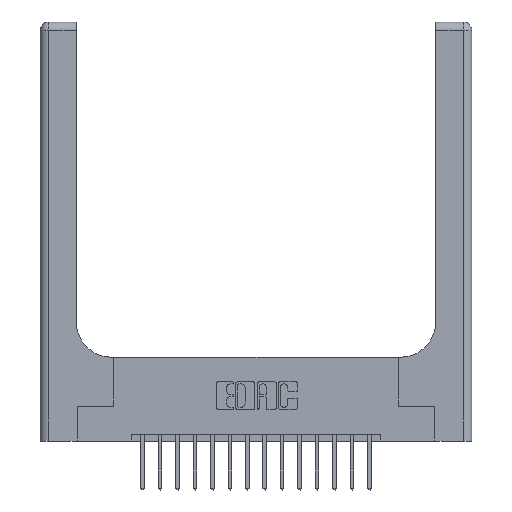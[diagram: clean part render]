
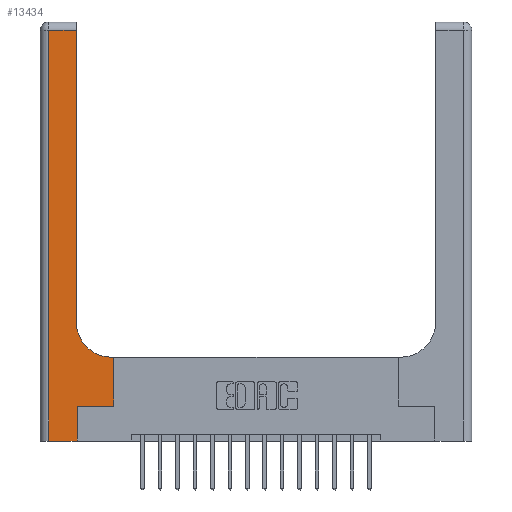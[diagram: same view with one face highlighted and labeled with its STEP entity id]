
A CAD part, top view. The second image highlights one B-rep face of the part: STEP entity #13434.
In plain terms, the highlighted planar face has unit normal (0, 0, 1).
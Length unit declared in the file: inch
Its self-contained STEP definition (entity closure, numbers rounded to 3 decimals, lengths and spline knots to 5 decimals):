
#68 = EDGE_CURVE ( 'NONE', #2373, #2701, #5165, .T. ) ;
#101 = ORIENTED_EDGE ( 'NONE', *, *, #17606, .T. ) ;
#243 = VECTOR ( 'NONE', #9647, 39.37008 ) ;
#904 = ORIENTED_EDGE ( 'NONE', *, *, #14326, .T. ) ;
#1054 = VECTOR ( 'NONE', #3244, 39.37008 ) ;
#1208 = CARTESIAN_POINT ( 'NONE',  ( 0.265, 0.25, 0.37 ) ) ;
#1668 = AXIS2_PLACEMENT_3D ( 'NONE', #18173, #14062, #3634 ) ;
#1882 = DIRECTION ( 'NONE',  ( 0., -1., 0. ) ) ;
#1957 = VERTEX_POINT ( 'NONE', #5199 ) ;
#2124 = DIRECTION ( 'NONE',  ( -1., 0., 0. ) ) ;
#2324 = CARTESIAN_POINT ( 'NONE',  ( 0.265, 0.25, 0.37 ) ) ;
#2373 = VERTEX_POINT ( 'NONE', #14361 ) ;
#2413 = ORIENTED_EDGE ( 'NONE', *, *, #68, .T. ) ;
#2423 = EDGE_LOOP ( 'NONE', ( #8129, #2413, #17395, #11864, #3161, #904, #18295, #101, #7175 ) ) ;
#2530 = EDGE_CURVE ( 'NONE', #5569, #14440, #15974, .T. ) ;
#2668 = CARTESIAN_POINT ( 'NONE',  ( 0.06, 2.94, 0.37 ) ) ;
#2701 = VERTEX_POINT ( 'NONE', #2668 ) ;
#2787 = EDGE_CURVE ( 'NONE', #10469, #5569, #15577, .T. ) ;
#2983 = VECTOR ( 'NONE', #2124, 39.37008 ) ;
#3161 = ORIENTED_EDGE ( 'NONE', *, *, #2530, .T. ) ;
#3244 = DIRECTION ( 'NONE',  ( 0., 1., 0. ) ) ;
#3326 = DIRECTION ( 'NONE',  ( -1., 0., 0. ) ) ;
#3634 = DIRECTION ( 'NONE',  ( -1., 0., 0. ) ) ;
#3943 = EDGE_CURVE ( 'NONE', #2701, #10469, #13005, .T. ) ;
#4748 = CARTESIAN_POINT ( 'NONE',  ( 0.528, 0.6, 0.37 ) ) ;
#4761 = CARTESIAN_POINT ( 'NONE',  ( 0.51, 0.85, 0.37 ) ) ;
#5066 = CIRCLE ( 'NONE', #15573, 0.25 ) ;
#5165 = LINE ( 'NONE', #16539, #2983 ) ;
#5199 = CARTESIAN_POINT ( 'NONE',  ( 0.26, 0.85, 0.37 ) ) ;
#5252 = CARTESIAN_POINT ( 'NONE',  ( 0.528, 0.25, 0.37 ) ) ;
#5287 = LINE ( 'NONE', #16749, #243 ) ;
#5569 = VERTEX_POINT ( 'NONE', #16203 ) ;
#5826 = CARTESIAN_POINT ( 'NONE',  ( 0.26, 0.6, 0.37 ) ) ;
#6036 = VERTEX_POINT ( 'NONE', #5252 ) ;
#6331 = DIRECTION ( 'NONE',  ( 0., 1., 0. ) ) ;
#6397 = FACE_OUTER_BOUND ( 'NONE', #2423, .T. ) ;
#6597 = VECTOR ( 'NONE', #1882, 39.37008 ) ;
#6974 = VERTEX_POINT ( 'NONE', #11674 ) ;
#7175 = ORIENTED_EDGE ( 'NONE', *, *, #18081, .T. ) ;
#8129 = ORIENTED_EDGE ( 'NONE', *, *, #15575, .T. ) ;
#8520 = CARTESIAN_POINT ( 'NONE',  ( 0., 0., 0.37 ) ) ;
#8633 = VECTOR ( 'NONE', #15851, 39.37008 ) ;
#8823 = CARTESIAN_POINT ( 'NONE',  ( 0.265, 0., 0.37 ) ) ;
#9131 = CARTESIAN_POINT ( 'NONE',  ( 0.528, 0.25, 0.37 ) ) ;
#9647 = DIRECTION ( 'NONE',  ( 0., 1., 0. ) ) ;
#10469 = VERTEX_POINT ( 'NONE', #11450 ) ;
#10629 = VERTEX_POINT ( 'NONE', #4748 ) ;
#11450 = CARTESIAN_POINT ( 'NONE',  ( 0.06, 0., 0.37 ) ) ;
#11674 = CARTESIAN_POINT ( 'NONE',  ( 0.51, 0.6, 0.37 ) ) ;
#11864 = ORIENTED_EDGE ( 'NONE', *, *, #2787, .T. ) ;
#11933 = VECTOR ( 'NONE', #15430, 39.37008 ) ;
#12794 = VECTOR ( 'NONE', #6331, 39.37008 ) ;
#12965 = EDGE_CURVE ( 'NONE', #6036, #10629, #16281, .T. ) ;
#13005 = LINE ( 'NONE', #14690, #6597 ) ;
#13434 = ADVANCED_FACE ( 'NONE', ( #6397 ), #18089, .F. ) ;
#14062 = DIRECTION ( 'NONE',  ( 0., 0., -1. ) ) ;
#14095 = LINE ( 'NONE', #2324, #11933 ) ;
#14326 = EDGE_CURVE ( 'NONE', #14440, #6036, #14095, .T. ) ;
#14350 = VECTOR ( 'NONE', #3326, 39.37008 ) ;
#14361 = CARTESIAN_POINT ( 'NONE',  ( 0.26, 2.94, 0.37 ) ) ;
#14440 = VERTEX_POINT ( 'NONE', #1208 ) ;
#14690 = CARTESIAN_POINT ( 'NONE',  ( 0.06, 3., 0.37 ) ) ;
#15430 = DIRECTION ( 'NONE',  ( 1., 0., 0. ) ) ;
#15573 = AXIS2_PLACEMENT_3D ( 'NONE', #4761, #16045, #16337 ) ;
#15575 = EDGE_CURVE ( 'NONE', #1957, #2373, #5287, .T. ) ;
#15577 = LINE ( 'NONE', #8520, #8633 ) ;
#15698 = LINE ( 'NONE', #5826, #14350 ) ;
#15851 = DIRECTION ( 'NONE',  ( 1., 0., 0. ) ) ;
#15974 = LINE ( 'NONE', #8823, #1054 ) ;
#16045 = DIRECTION ( 'NONE',  ( 0., 0., -1. ) ) ;
#16203 = CARTESIAN_POINT ( 'NONE',  ( 0.265, 0., 0.37 ) ) ;
#16281 = LINE ( 'NONE', #9131, #12794 ) ;
#16337 = DIRECTION ( 'NONE',  ( 1., 0., 0. ) ) ;
#16539 = CARTESIAN_POINT ( 'NONE',  ( 0., 2.94, 0.37 ) ) ;
#16749 = CARTESIAN_POINT ( 'NONE',  ( 0.26, 3., 0.37 ) ) ;
#17395 = ORIENTED_EDGE ( 'NONE', *, *, #3943, .T. ) ;
#17606 = EDGE_CURVE ( 'NONE', #10629, #6974, #15698, .T. ) ;
#18081 = EDGE_CURVE ( 'NONE', #6974, #1957, #5066, .T. ) ;
#18089 = PLANE ( 'NONE',  #1668 ) ;
#18173 = CARTESIAN_POINT ( 'NONE',  ( 0., 3., 0.37 ) ) ;
#18295 = ORIENTED_EDGE ( 'NONE', *, *, #12965, .T. ) ;
